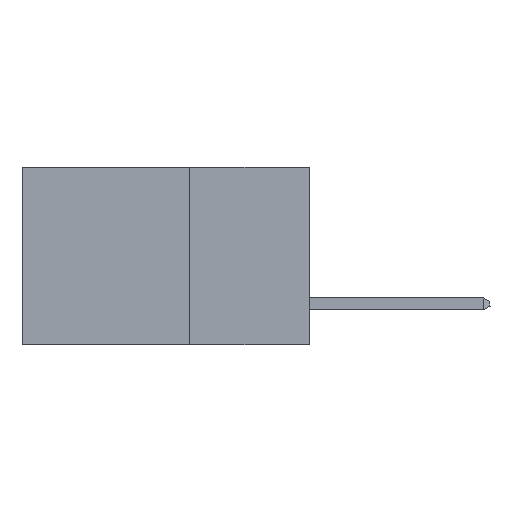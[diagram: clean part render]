
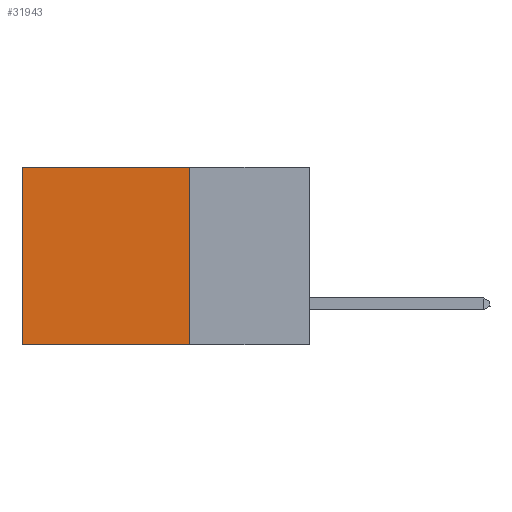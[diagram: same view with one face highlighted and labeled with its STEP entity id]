
A CAD part, left-side view. The second image highlights one B-rep face of the part: STEP entity #31943.
In plain terms, the highlighted planar face has unit normal (-1, 0, 0).
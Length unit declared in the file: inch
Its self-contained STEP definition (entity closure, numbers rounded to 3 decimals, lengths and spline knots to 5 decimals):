
#41 = DIRECTION ( 'NONE',  ( 0., 1., 0. ) ) ;
#2545 = CARTESIAN_POINT ( 'NONE',  ( 0.2875, 0.6, -0.37 ) ) ;
#5830 = ORIENTED_EDGE ( 'NONE', *, *, #31538, .T. ) ;
#7534 = DIRECTION ( 'NONE',  ( 0., 0., -1. ) ) ;
#8011 = DIRECTION ( 'NONE',  ( 0., 1., 0. ) ) ;
#9955 = DIRECTION ( 'NONE',  ( 1., 0., 0. ) ) ;
#10102 = ORIENTED_EDGE ( 'NONE', *, *, #20549, .F. ) ;
#10712 = EDGE_LOOP ( 'NONE', ( #37526, #12734, #10102, #5830 ) ) ;
#11578 = AXIS2_PLACEMENT_3D ( 'NONE', #43812, #9955, #28347 ) ;
#12037 = VERTEX_POINT ( 'NONE', #30090 ) ;
#12734 = ORIENTED_EDGE ( 'NONE', *, *, #44696, .F. ) ;
#13710 = PLANE ( 'NONE',  #11578 ) ;
#15538 = DIRECTION ( 'NONE',  ( 0., 0., -1. ) ) ;
#17282 = VERTEX_POINT ( 'NONE', #2545 ) ;
#20549 = EDGE_CURVE ( 'NONE', #31765, #21641, #21631, .T. ) ;
#21631 = LINE ( 'NONE', #45815, #32769 ) ;
#21641 = VERTEX_POINT ( 'NONE', #41634 ) ;
#25232 = LINE ( 'NONE', #26571, #39850 ) ;
#26571 = CARTESIAN_POINT ( 'NONE',  ( 0.2875, 0.25, 0. ) ) ;
#27545 = VECTOR ( 'NONE', #7534, 39.37008 ) ;
#28347 = DIRECTION ( 'NONE',  ( 0., 0., -1. ) ) ;
#29430 = VECTOR ( 'NONE', #8011, 39.37008 ) ;
#30090 = CARTESIAN_POINT ( 'NONE',  ( 0.2875, 0.6, 0. ) ) ;
#30323 = CARTESIAN_POINT ( 'NONE',  ( 0.2875, 0.25, -0.37 ) ) ;
#31533 = EDGE_CURVE ( 'NONE', #12037, #17282, #46195, .T. ) ;
#31538 = EDGE_CURVE ( 'NONE', #31765, #12037, #25232, .T. ) ;
#31765 = VERTEX_POINT ( 'NONE', #35208 ) ;
#31943 = ADVANCED_FACE ( 'NONE', ( #33933 ), #13710, .F. ) ;
#32769 = VECTOR ( 'NONE', #15538, 39.37008 ) ;
#33933 = FACE_OUTER_BOUND ( 'NONE', #10712, .T. ) ;
#35208 = CARTESIAN_POINT ( 'NONE',  ( 0.2875, 0.25, 0. ) ) ;
#37215 = CARTESIAN_POINT ( 'NONE',  ( 0.2875, 0.6, 0. ) ) ;
#37526 = ORIENTED_EDGE ( 'NONE', *, *, #31533, .T. ) ;
#39850 = VECTOR ( 'NONE', #41, 39.37008 ) ;
#41122 = LINE ( 'NONE', #30323, #29430 ) ;
#41634 = CARTESIAN_POINT ( 'NONE',  ( 0.2875, 0.25, -0.37 ) ) ;
#43812 = CARTESIAN_POINT ( 'NONE',  ( 0.2875, 0.25, 0. ) ) ;
#44696 = EDGE_CURVE ( 'NONE', #21641, #17282, #41122, .T. ) ;
#45815 = CARTESIAN_POINT ( 'NONE',  ( 0.2875, 0.25, 0. ) ) ;
#46195 = LINE ( 'NONE', #37215, #27545 ) ;
